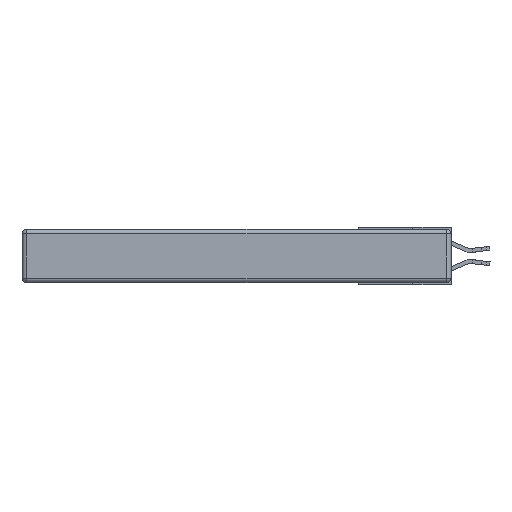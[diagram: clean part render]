
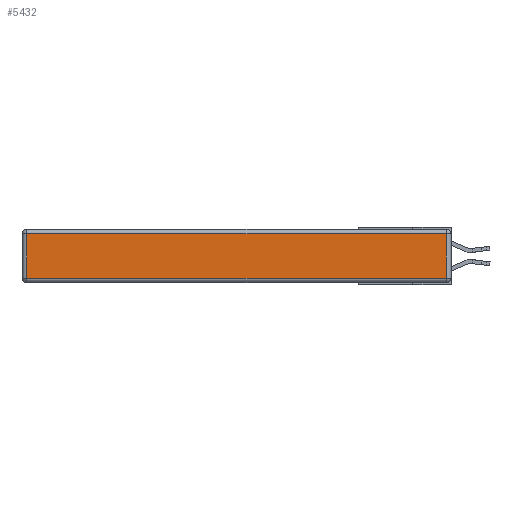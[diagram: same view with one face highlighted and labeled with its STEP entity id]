
A CAD part, left-side view. The second image highlights one B-rep face of the part: STEP entity #5432.
In plain terms, the highlighted planar face has unit normal (-1, 0, 0).
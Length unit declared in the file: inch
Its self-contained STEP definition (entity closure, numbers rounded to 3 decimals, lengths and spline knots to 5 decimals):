
#897 = VECTOR ( 'NONE', #12606, 39.37008 ) ;
#1389 = EDGE_LOOP ( 'NONE', ( #4509, #13766, #2571, #11760 ) ) ;
#1839 = EDGE_CURVE ( 'NONE', #12204, #11911, #13846, .T. ) ;
#2061 = VECTOR ( 'NONE', #7891, 39.37008 ) ;
#2285 = CARTESIAN_POINT ( 'NONE',  ( 0., 0.03, -0.03 ) ) ;
#2500 = VECTOR ( 'NONE', #12458, 39.37008 ) ;
#2571 = ORIENTED_EDGE ( 'NONE', *, *, #6268, .T. ) ;
#2601 = CARTESIAN_POINT ( 'NONE',  ( 0., 0.03, -0.313 ) ) ;
#2613 = VERTEX_POINT ( 'NONE', #2285 ) ;
#3645 = CARTESIAN_POINT ( 'NONE',  ( 0., 0.03, -0.343 ) ) ;
#4433 = CARTESIAN_POINT ( 'NONE',  ( 0., 0., -0.343 ) ) ;
#4509 = ORIENTED_EDGE ( 'NONE', *, *, #1839, .T. ) ;
#5149 = EDGE_CURVE ( 'NONE', #11911, #2613, #12891, .T. ) ;
#5255 = VECTOR ( 'NONE', #12951, 39.37008 ) ;
#5432 = ADVANCED_FACE ( 'NONE', ( #14093 ), #9574, .T. ) ;
#5719 = CARTESIAN_POINT ( 'NONE',  ( 0., 2.72, -0.313 ) ) ;
#5853 = CARTESIAN_POINT ( 'NONE',  ( 0., 0., -0.313 ) ) ;
#6243 = CARTESIAN_POINT ( 'NONE',  ( 0., 2.75, -0.03 ) ) ;
#6268 = EDGE_CURVE ( 'NONE', #2613, #10799, #13707, .T. ) ;
#7891 = DIRECTION ( 'NONE',  ( 0., -1., 0. ) ) ;
#9574 = PLANE ( 'NONE',  #12791 ) ;
#10201 = DIRECTION ( 'NONE',  ( 0., 0., 1. ) ) ;
#10799 = VERTEX_POINT ( 'NONE', #13855 ) ;
#10827 = LINE ( 'NONE', #14319, #2500 ) ;
#11760 = ORIENTED_EDGE ( 'NONE', *, *, #12999, .T. ) ;
#11911 = VERTEX_POINT ( 'NONE', #2601 ) ;
#12204 = VERTEX_POINT ( 'NONE', #5719 ) ;
#12458 = DIRECTION ( 'NONE',  ( 0., 0., -1. ) ) ;
#12606 = DIRECTION ( 'NONE',  ( 0., 0., 1. ) ) ;
#12791 = AXIS2_PLACEMENT_3D ( 'NONE', #4433, #13381, #10201 ) ;
#12891 = LINE ( 'NONE', #3645, #897 ) ;
#12951 = DIRECTION ( 'NONE',  ( 0., 1., 0. ) ) ;
#12999 = EDGE_CURVE ( 'NONE', #10799, #12204, #10827, .T. ) ;
#13381 = DIRECTION ( 'NONE',  ( -1., 0., 0. ) ) ;
#13707 = LINE ( 'NONE', #6243, #5255 ) ;
#13766 = ORIENTED_EDGE ( 'NONE', *, *, #5149, .T. ) ;
#13846 = LINE ( 'NONE', #5853, #2061 ) ;
#13855 = CARTESIAN_POINT ( 'NONE',  ( 0., 2.72, -0.03 ) ) ;
#14093 = FACE_OUTER_BOUND ( 'NONE', #1389, .T. ) ;
#14319 = CARTESIAN_POINT ( 'NONE',  ( 0., 2.72, -0.343 ) ) ;
